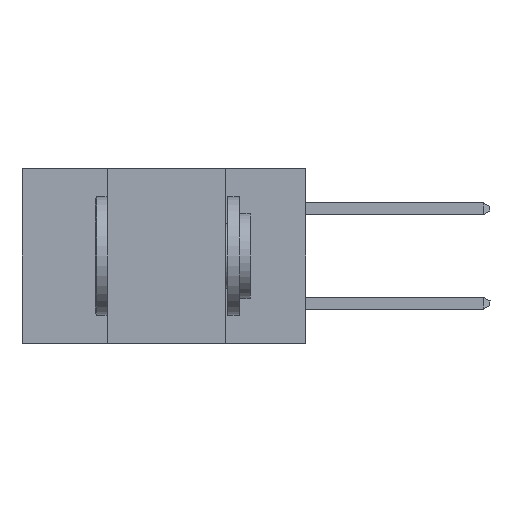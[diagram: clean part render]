
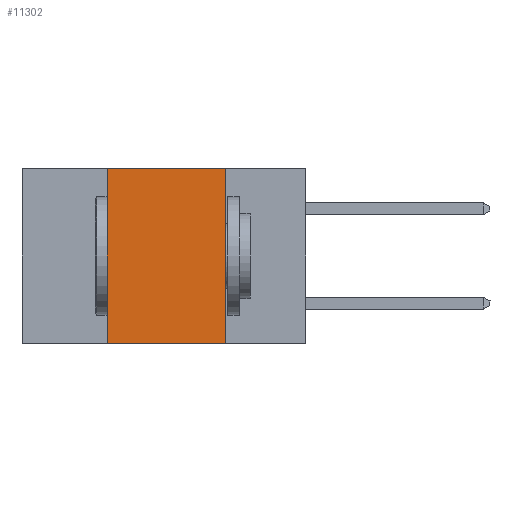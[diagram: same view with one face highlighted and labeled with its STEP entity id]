
A CAD part, left-side view. The second image highlights one B-rep face of the part: STEP entity #11302.
In plain terms, the highlighted planar face has unit normal (-1, 0, 0).
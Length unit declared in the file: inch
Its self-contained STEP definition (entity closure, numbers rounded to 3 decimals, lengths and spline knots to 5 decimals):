
#404 = DIRECTION ( 'NONE',  ( 0., -1., 0. ) ) ;
#630 = CARTESIAN_POINT ( 'NONE',  ( 0., 0.17, 0. ) ) ;
#1156 = AXIS2_PLACEMENT_3D ( 'NONE', #13068, #11907, #11957 ) ;
#2053 = VECTOR ( 'NONE', #11688, 39.37008 ) ;
#2319 = PLANE ( 'NONE',  #1156 ) ;
#2461 = VECTOR ( 'NONE', #404, 39.37008 ) ;
#2844 = VERTEX_POINT ( 'NONE', #630 ) ;
#3072 = VERTEX_POINT ( 'NONE', #9043 ) ;
#3175 = CARTESIAN_POINT ( 'NONE',  ( 0., 0.17, 0. ) ) ;
#3367 = EDGE_CURVE ( 'NONE', #2844, #3072, #7113, .T. ) ;
#3490 = DIRECTION ( 'NONE',  ( 0., 0., 1. ) ) ;
#3544 = VERTEX_POINT ( 'NONE', #13087 ) ;
#4254 = DIRECTION ( 'NONE',  ( 0., -1., 0. ) ) ;
#4860 = CARTESIAN_POINT ( 'NONE',  ( 0., 0.42, -0.37 ) ) ;
#7113 = LINE ( 'NONE', #3175, #2053 ) ;
#7820 = ORIENTED_EDGE ( 'NONE', *, *, #3367, .F. ) ;
#7848 = LINE ( 'NONE', #13165, #10856 ) ;
#8146 = LINE ( 'NONE', #9620, #9478 ) ;
#8171 = LINE ( 'NONE', #13352, #2461 ) ;
#8372 = VERTEX_POINT ( 'NONE', #4860 ) ;
#8588 = ORIENTED_EDGE ( 'NONE', *, *, #11774, .T. ) ;
#9043 = CARTESIAN_POINT ( 'NONE',  ( 0., 0.17, -0.37 ) ) ;
#9354 = ORIENTED_EDGE ( 'NONE', *, *, #11439, .F. ) ;
#9478 = VECTOR ( 'NONE', #4254, 39.37008 ) ;
#9620 = CARTESIAN_POINT ( 'NONE',  ( 0., 0.6, 0. ) ) ;
#9843 = FACE_OUTER_BOUND ( 'NONE', #12791, .T. ) ;
#10856 = VECTOR ( 'NONE', #3490, 39.37008 ) ;
#11302 = ADVANCED_FACE ( 'NONE', ( #9843 ), #2319, .F. ) ;
#11439 = EDGE_CURVE ( 'NONE', #8372, #3544, #7848, .T. ) ;
#11688 = DIRECTION ( 'NONE',  ( 0., 0., -1. ) ) ;
#11774 = EDGE_CURVE ( 'NONE', #8372, #3072, #8171, .T. ) ;
#11907 = DIRECTION ( 'NONE',  ( 1., 0., 0. ) ) ;
#11957 = DIRECTION ( 'NONE',  ( 0., 0., -1. ) ) ;
#12499 = EDGE_CURVE ( 'NONE', #3544, #2844, #8146, .T. ) ;
#12511 = ORIENTED_EDGE ( 'NONE', *, *, #12499, .F. ) ;
#12791 = EDGE_LOOP ( 'NONE', ( #7820, #12511, #9354, #8588 ) ) ;
#13068 = CARTESIAN_POINT ( 'NONE',  ( 0., 0.6, 0. ) ) ;
#13087 = CARTESIAN_POINT ( 'NONE',  ( 0., 0.42, 0. ) ) ;
#13165 = CARTESIAN_POINT ( 'NONE',  ( 0., 0.42, 0. ) ) ;
#13352 = CARTESIAN_POINT ( 'NONE',  ( 0., 0.6, -0.37 ) ) ;
